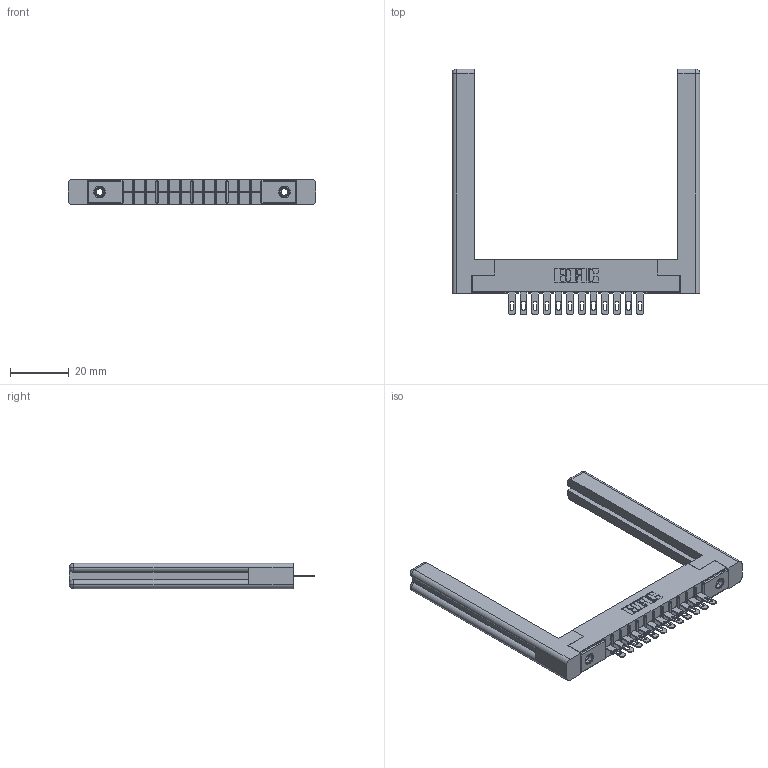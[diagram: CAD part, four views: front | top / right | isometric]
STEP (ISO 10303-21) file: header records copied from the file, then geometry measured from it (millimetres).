
FILE_DESCRIPTION (( 'STEP AP203' ), '1' );
FILE_NAME ('306-012-400-158.STEP', '2020-09-21T17:02:13', ( '' ), ( '' ), 'SwSTEP 2.0', 'SolidWorks 2020', '' );
FILE_SCHEMA (( 'CONFIG_CONTROL_DESIGN' ));
Length unit declared in the file: inch
Products named in the file (5): 345-250-001_345-250-001-102; 306 Part_.156 Dia; 307-220-058; 306-290-001_100; 306-012-400-158
Assembly tree (17 placements, depth 2):
  306-012-400-158
    306 Part_.156 Dia
    306-290-001_100  x12
    345-250-001_345-250-001-102  x2
    307-220-058  x2
Bounding box: 84.18 x 83.52 x 8.71 mm (x, y, z)
Volume: 13393.5 mm3; surface area: 13673.5 mm2
Topology: 17 solids, 17 shells, 1170 faces, 3250 edges, 2088 vertices
Faces by surface type: plane 752, cylinder 346, sphere 48, cone 12, torus 12
Entity records: 17874 total; most frequent: CARTESIAN_POINT 3006, DIRECTION 2923, ORIENTED_EDGE 2918, EDGE_CURVE 1459, VECTOR 1117, LINE 1117, VERTEX_POINT 932, AXIS2_PLACEMENT_3D 903
